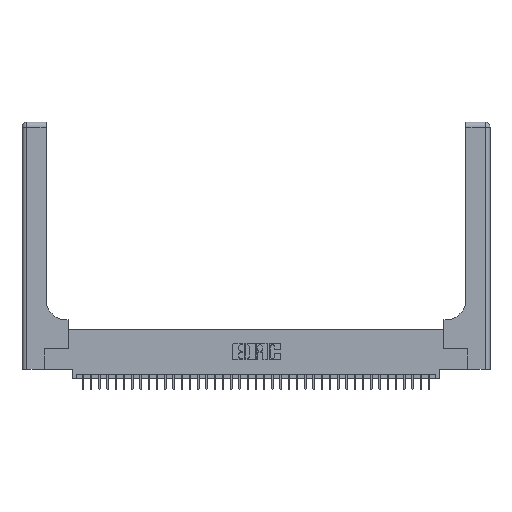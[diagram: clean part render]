
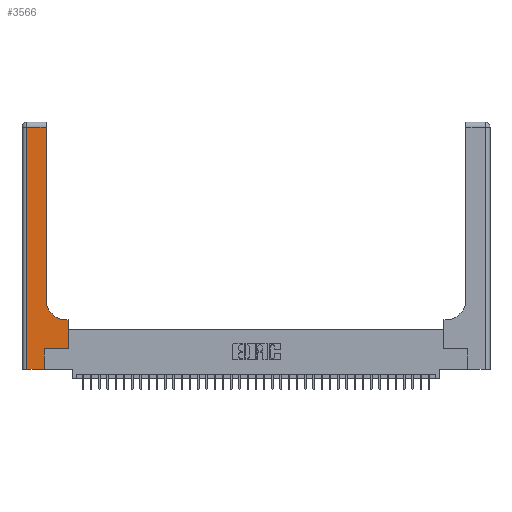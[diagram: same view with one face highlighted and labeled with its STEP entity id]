
A CAD part, top view. The second image highlights one B-rep face of the part: STEP entity #3566.
In plain terms, the highlighted planar face has unit normal (0, 0, 1).
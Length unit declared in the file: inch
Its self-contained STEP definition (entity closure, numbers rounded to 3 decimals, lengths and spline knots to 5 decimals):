
#453 = LINE ( 'NONE', #15252, #34962 ) ;
#619 = EDGE_CURVE ( 'NONE', #1675, #30091, #13060, .T. ) ;
#1489 = LINE ( 'NONE', #13469, #16252 ) ;
#1675 = VERTEX_POINT ( 'NONE', #16020 ) ;
#3566 = ADVANCED_FACE ( 'NONE', ( #11884 ), #38793, .F. ) ;
#3766 = AXIS2_PLACEMENT_3D ( 'NONE', #36385, #29871, #20772 ) ;
#4197 = CARTESIAN_POINT ( 'NONE',  ( 0.5585, 0.25, 0.37 ) ) ;
#4710 = VECTOR ( 'NONE', #13442, 39.37008 ) ;
#6896 = ORIENTED_EDGE ( 'NONE', *, *, #26688, .T. ) ;
#6977 = CARTESIAN_POINT ( 'NONE',  ( 0.2915, 3., 0.37 ) ) ;
#7201 = EDGE_CURVE ( 'NONE', #32475, #28205, #20965, .T. ) ;
#7282 = DIRECTION ( 'NONE',  ( -1., 0., 0. ) ) ;
#9104 = DIRECTION ( 'NONE',  ( -1., 0., 0. ) ) ;
#9828 = DIRECTION ( 'NONE',  ( 0., 1., 0. ) ) ;
#9984 = VECTOR ( 'NONE', #30067, 39.37008 ) ;
#10016 = CIRCLE ( 'NONE', #3766, 0.25 ) ;
#10216 = LINE ( 'NONE', #24906, #10945 ) ;
#10945 = VECTOR ( 'NONE', #9828, 39.37008 ) ;
#11073 = VERTEX_POINT ( 'NONE', #36538 ) ;
#11081 = DIRECTION ( 'NONE',  ( -1., 0., 0. ) ) ;
#11706 = AXIS2_PLACEMENT_3D ( 'NONE', #29335, #32917, #11081 ) ;
#11884 = FACE_OUTER_BOUND ( 'NONE', #28450, .T. ) ;
#12059 = LINE ( 'NONE', #24172, #30498 ) ;
#12369 = VERTEX_POINT ( 'NONE', #15053 ) ;
#12783 = EDGE_CURVE ( 'NONE', #11073, #1675, #10016, .T. ) ;
#12854 = DIRECTION ( 'NONE',  ( 0., 1., 0. ) ) ;
#13060 = LINE ( 'NONE', #6977, #4710 ) ;
#13442 = DIRECTION ( 'NONE',  ( 0., 1., 0. ) ) ;
#13469 = CARTESIAN_POINT ( 'NONE',  ( 0.269, 0.25, 0.37 ) ) ;
#14246 = CARTESIAN_POINT ( 'NONE',  ( 0.2915, 2.94, 0.37 ) ) ;
#14344 = CARTESIAN_POINT ( 'NONE',  ( 0.06, 2.94, 0.37 ) ) ;
#15053 = CARTESIAN_POINT ( 'NONE',  ( 0.269, 0.25, 0.37 ) ) ;
#15252 = CARTESIAN_POINT ( 'NONE',  ( 0., 0., 0.37 ) ) ;
#16020 = CARTESIAN_POINT ( 'NONE',  ( 0.2915, 0.85, 0.37 ) ) ;
#16252 = VECTOR ( 'NONE', #29168, 39.37008 ) ;
#17736 = ORIENTED_EDGE ( 'NONE', *, *, #7201, .T. ) ;
#17996 = CARTESIAN_POINT ( 'NONE',  ( 0.06, 3., 0.37 ) ) ;
#18278 = VECTOR ( 'NONE', #12854, 39.37008 ) ;
#18829 = EDGE_CURVE ( 'NONE', #28205, #22965, #453, .T. ) ;
#19819 = VECTOR ( 'NONE', #7282, 39.37008 ) ;
#19992 = ORIENTED_EDGE ( 'NONE', *, *, #12783, .T. ) ;
#20772 = DIRECTION ( 'NONE',  ( 1., 0., 0. ) ) ;
#20965 = LINE ( 'NONE', #17996, #9984 ) ;
#21211 = DIRECTION ( 'NONE',  ( 1., 0., 0. ) ) ;
#21407 = CARTESIAN_POINT ( 'NONE',  ( 0.5585, 0.6, 0.37 ) ) ;
#21894 = ORIENTED_EDGE ( 'NONE', *, *, #37577, .T. ) ;
#22541 = LINE ( 'NONE', #31094, #19819 ) ;
#22876 = CARTESIAN_POINT ( 'NONE',  ( 0.5585, 0.25, 0.37 ) ) ;
#22965 = VERTEX_POINT ( 'NONE', #25047 ) ;
#24172 = CARTESIAN_POINT ( 'NONE',  ( 0.2915, 0.6, 0.37 ) ) ;
#24906 = CARTESIAN_POINT ( 'NONE',  ( 0.269, 0., 0.37 ) ) ;
#25047 = CARTESIAN_POINT ( 'NONE',  ( 0.269, 0., 0.37 ) ) ;
#25198 = ORIENTED_EDGE ( 'NONE', *, *, #28271, .T. ) ;
#26688 = EDGE_CURVE ( 'NONE', #12369, #35686, #1489, .T. ) ;
#27139 = ORIENTED_EDGE ( 'NONE', *, *, #619, .T. ) ;
#28205 = VERTEX_POINT ( 'NONE', #33528 ) ;
#28271 = EDGE_CURVE ( 'NONE', #35686, #37380, #31128, .T. ) ;
#28450 = EDGE_LOOP ( 'NONE', ( #27139, #21894, #17736, #34228, #34192, #6896, #25198, #34989, #19992 ) ) ;
#29168 = DIRECTION ( 'NONE',  ( 1., 0., 0. ) ) ;
#29335 = CARTESIAN_POINT ( 'NONE',  ( 0., 3., 0.37 ) ) ;
#29871 = DIRECTION ( 'NONE',  ( 0., 0., -1. ) ) ;
#30067 = DIRECTION ( 'NONE',  ( 0., -1., 0. ) ) ;
#30091 = VERTEX_POINT ( 'NONE', #14246 ) ;
#30498 = VECTOR ( 'NONE', #9104, 39.37008 ) ;
#31094 = CARTESIAN_POINT ( 'NONE',  ( 0., 2.94, 0.37 ) ) ;
#31128 = LINE ( 'NONE', #4197, #18278 ) ;
#32475 = VERTEX_POINT ( 'NONE', #14344 ) ;
#32917 = DIRECTION ( 'NONE',  ( 0., 0., -1. ) ) ;
#33528 = CARTESIAN_POINT ( 'NONE',  ( 0.06, 0., 0.37 ) ) ;
#34192 = ORIENTED_EDGE ( 'NONE', *, *, #37975, .T. ) ;
#34228 = ORIENTED_EDGE ( 'NONE', *, *, #18829, .T. ) ;
#34325 = EDGE_CURVE ( 'NONE', #37380, #11073, #12059, .T. ) ;
#34962 = VECTOR ( 'NONE', #21211, 39.37008 ) ;
#34989 = ORIENTED_EDGE ( 'NONE', *, *, #34325, .T. ) ;
#35686 = VERTEX_POINT ( 'NONE', #22876 ) ;
#36385 = CARTESIAN_POINT ( 'NONE',  ( 0.5415, 0.85, 0.37 ) ) ;
#36538 = CARTESIAN_POINT ( 'NONE',  ( 0.5415, 0.6, 0.37 ) ) ;
#37380 = VERTEX_POINT ( 'NONE', #21407 ) ;
#37577 = EDGE_CURVE ( 'NONE', #30091, #32475, #22541, .T. ) ;
#37975 = EDGE_CURVE ( 'NONE', #22965, #12369, #10216, .T. ) ;
#38793 = PLANE ( 'NONE',  #11706 ) ;
